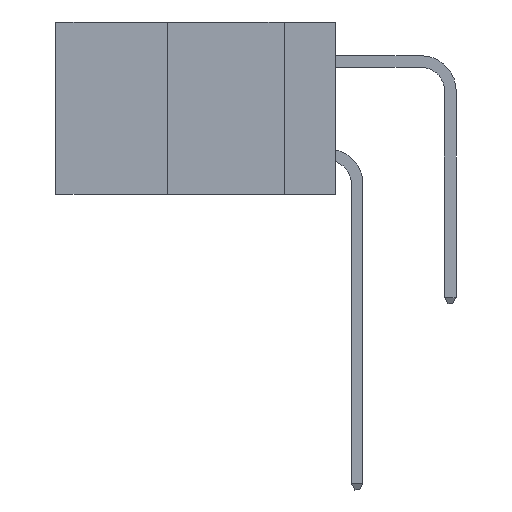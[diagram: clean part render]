
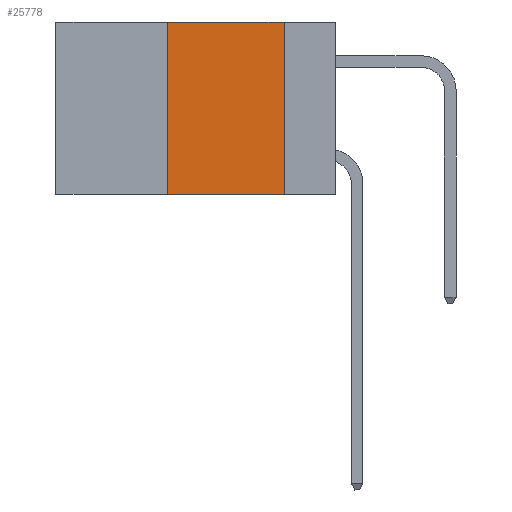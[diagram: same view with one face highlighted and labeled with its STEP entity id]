
A CAD part, left-side view. The second image highlights one B-rep face of the part: STEP entity #25778.
In plain terms, the highlighted planar face has unit normal (-1, 0, 0).
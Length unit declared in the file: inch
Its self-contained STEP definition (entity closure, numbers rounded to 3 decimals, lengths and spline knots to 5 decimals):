
#1291 = CARTESIAN_POINT ( 'NONE',  ( 0., 0.36, 0. ) ) ;
#2390 = CARTESIAN_POINT ( 'NONE',  ( 0., 0.6, 0. ) ) ;
#4680 = VERTEX_POINT ( 'NONE', #35212 ) ;
#5417 = ORIENTED_EDGE ( 'NONE', *, *, #24021, .F. ) ;
#7567 = LINE ( 'NONE', #2390, #43488 ) ;
#7796 = DIRECTION ( 'NONE',  ( 1., 0., 0. ) ) ;
#8672 = AXIS2_PLACEMENT_3D ( 'NONE', #24794, #7796, #38455 ) ;
#9229 = EDGE_CURVE ( 'NONE', #42448, #30760, #7567, .T. ) ;
#10119 = CARTESIAN_POINT ( 'NONE',  ( 0., 0.11, 0. ) ) ;
#12159 = LINE ( 'NONE', #42409, #23254 ) ;
#12184 = CARTESIAN_POINT ( 'NONE',  ( 0., 0.6, -0.37 ) ) ;
#12494 = CARTESIAN_POINT ( 'NONE',  ( 0., 0.36, -0.37 ) ) ;
#14929 = PLANE ( 'NONE',  #8672 ) ;
#15307 = ORIENTED_EDGE ( 'NONE', *, *, #28068, .F. ) ;
#16239 = CARTESIAN_POINT ( 'NONE',  ( 0., 0.11, 0. ) ) ;
#18050 = ORIENTED_EDGE ( 'NONE', *, *, #9229, .F. ) ;
#22933 = VECTOR ( 'NONE', #29507, 39.37008 ) ;
#23254 = VECTOR ( 'NONE', #25465, 39.37008 ) ;
#24021 = EDGE_CURVE ( 'NONE', #37085, #42448, #12159, .T. ) ;
#24324 = ORIENTED_EDGE ( 'NONE', *, *, #35324, .T. ) ;
#24766 = FACE_OUTER_BOUND ( 'NONE', #29024, .T. ) ;
#24794 = CARTESIAN_POINT ( 'NONE',  ( 0., 0.6, 0. ) ) ;
#25465 = DIRECTION ( 'NONE',  ( 0., 0., 1. ) ) ;
#25778 = ADVANCED_FACE ( 'NONE', ( #24766 ), #14929, .F. ) ;
#28068 = EDGE_CURVE ( 'NONE', #30760, #4680, #41939, .T. ) ;
#29024 = EDGE_LOOP ( 'NONE', ( #15307, #18050, #5417, #24324 ) ) ;
#29431 = DIRECTION ( 'NONE',  ( 0., -1., 0. ) ) ;
#29507 = DIRECTION ( 'NONE',  ( 0., 0., -1. ) ) ;
#29533 = LINE ( 'NONE', #12184, #32621 ) ;
#30760 = VERTEX_POINT ( 'NONE', #10119 ) ;
#32621 = VECTOR ( 'NONE', #35751, 39.37008 ) ;
#35212 = CARTESIAN_POINT ( 'NONE',  ( 0., 0.11, -0.37 ) ) ;
#35324 = EDGE_CURVE ( 'NONE', #37085, #4680, #29533, .T. ) ;
#35751 = DIRECTION ( 'NONE',  ( 0., -1., 0. ) ) ;
#37085 = VERTEX_POINT ( 'NONE', #12494 ) ;
#38455 = DIRECTION ( 'NONE',  ( 0., 0., -1. ) ) ;
#41939 = LINE ( 'NONE', #16239, #22933 ) ;
#42409 = CARTESIAN_POINT ( 'NONE',  ( 0., 0.36, 0. ) ) ;
#42448 = VERTEX_POINT ( 'NONE', #1291 ) ;
#43488 = VECTOR ( 'NONE', #29431, 39.37008 ) ;
